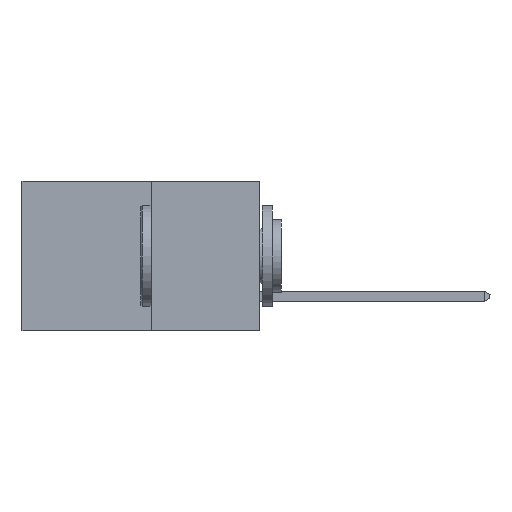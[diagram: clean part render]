
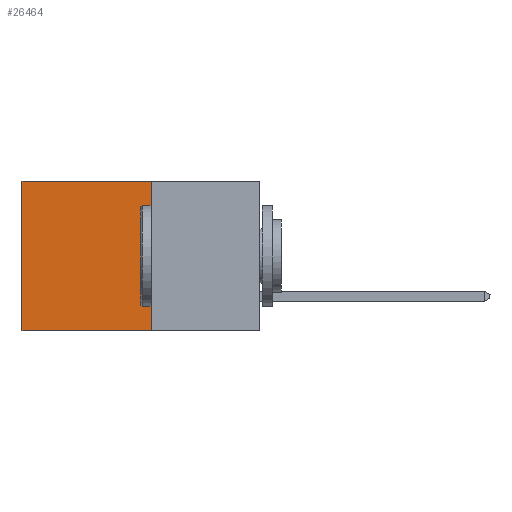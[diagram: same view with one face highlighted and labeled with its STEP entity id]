
A CAD part, left-side view. The second image highlights one B-rep face of the part: STEP entity #26464.
In plain terms, the highlighted planar face has unit normal (-1, 0, 0).
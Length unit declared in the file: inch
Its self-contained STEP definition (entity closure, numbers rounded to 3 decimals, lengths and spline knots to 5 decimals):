
#234 = CARTESIAN_POINT ( 'NONE',  ( 0.277, 0.27, -0.37 ) ) ;
#616 = ORIENTED_EDGE ( 'NONE', *, *, #7019, .F. ) ;
#1710 = EDGE_CURVE ( 'NONE', #26671, #8362, #25868, .T. ) ;
#1989 = DIRECTION ( 'NONE',  ( 0., 0., -1. ) ) ;
#2706 = FACE_OUTER_BOUND ( 'NONE', #25061, .T. ) ;
#5556 = CARTESIAN_POINT ( 'NONE',  ( 0.277, 0.27, 0. ) ) ;
#5854 = DIRECTION ( 'NONE',  ( 0., 0., -1. ) ) ;
#7019 = EDGE_CURVE ( 'NONE', #20395, #13262, #28560, .T. ) ;
#8362 = VERTEX_POINT ( 'NONE', #27193 ) ;
#9747 = CARTESIAN_POINT ( 'NONE',  ( 0.277, 0.59, 0. ) ) ;
#10955 = VECTOR ( 'NONE', #5854, 39.37008 ) ;
#10958 = AXIS2_PLACEMENT_3D ( 'NONE', #20631, #16112, #1989 ) ;
#12701 = CARTESIAN_POINT ( 'NONE',  ( 0.277, 0.27, 0. ) ) ;
#12705 = CARTESIAN_POINT ( 'NONE',  ( 0.277, 0.27, -0.37 ) ) ;
#12802 = VECTOR ( 'NONE', #14933, 39.37008 ) ;
#13262 = VERTEX_POINT ( 'NONE', #12705 ) ;
#14245 = LINE ( 'NONE', #5556, #12802 ) ;
#14933 = DIRECTION ( 'NONE',  ( 0., 1., 0. ) ) ;
#16112 = DIRECTION ( 'NONE',  ( 1., 0., 0. ) ) ;
#16380 = ORIENTED_EDGE ( 'NONE', *, *, #26663, .F. ) ;
#16403 = CARTESIAN_POINT ( 'NONE',  ( 0.277, 0.27, -0.37 ) ) ;
#18301 = PLANE ( 'NONE',  #10958 ) ;
#19735 = VECTOR ( 'NONE', #26862, 39.37008 ) ;
#20395 = VERTEX_POINT ( 'NONE', #12701 ) ;
#20631 = CARTESIAN_POINT ( 'NONE',  ( 0.277, 0.27, -0.37 ) ) ;
#24853 = ORIENTED_EDGE ( 'NONE', *, *, #1710, .T. ) ;
#25061 = EDGE_LOOP ( 'NONE', ( #24853, #16380, #616, #26662 ) ) ;
#25515 = EDGE_CURVE ( 'NONE', #20395, #26671, #14245, .T. ) ;
#25831 = DIRECTION ( 'NONE',  ( 0., 1., 0. ) ) ;
#25868 = LINE ( 'NONE', #27130, #19735 ) ;
#26464 = ADVANCED_FACE ( 'NONE', ( #2706 ), #18301, .F. ) ;
#26662 = ORIENTED_EDGE ( 'NONE', *, *, #25515, .T. ) ;
#26663 = EDGE_CURVE ( 'NONE', #13262, #8362, #27792, .T. ) ;
#26671 = VERTEX_POINT ( 'NONE', #9747 ) ;
#26862 = DIRECTION ( 'NONE',  ( 0., 0., -1. ) ) ;
#27105 = VECTOR ( 'NONE', #25831, 39.37008 ) ;
#27130 = CARTESIAN_POINT ( 'NONE',  ( 0.277, 0.59, -0.37 ) ) ;
#27193 = CARTESIAN_POINT ( 'NONE',  ( 0.277, 0.59, -0.37 ) ) ;
#27792 = LINE ( 'NONE', #234, #27105 ) ;
#28560 = LINE ( 'NONE', #16403, #10955 ) ;
